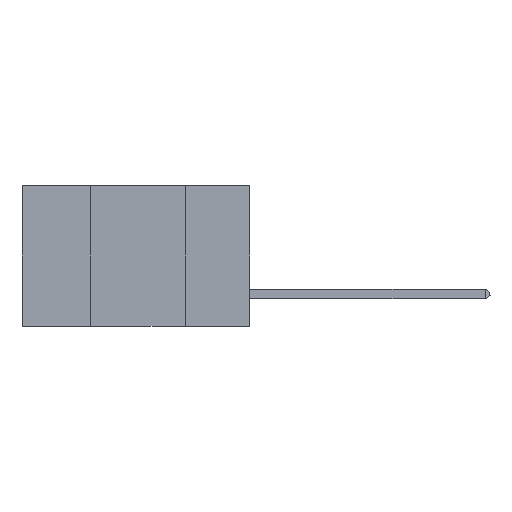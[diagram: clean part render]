
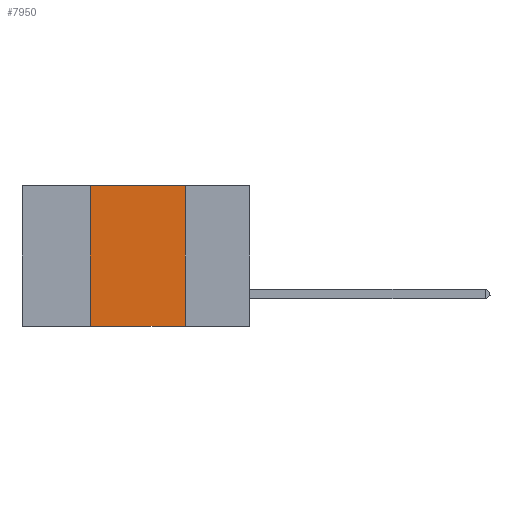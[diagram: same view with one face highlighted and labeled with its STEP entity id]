
A CAD part, left-side view. The second image highlights one B-rep face of the part: STEP entity #7950.
In plain terms, the highlighted planar face has unit normal (-1, 0, 0).
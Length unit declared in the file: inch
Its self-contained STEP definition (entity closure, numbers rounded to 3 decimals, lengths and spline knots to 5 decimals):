
#810 = VECTOR ( 'NONE', #14395, 39.37008 ) ;
#1160 = ORIENTED_EDGE ( 'NONE', *, *, #2776, .F. ) ;
#1202 = EDGE_CURVE ( 'NONE', #4131, #8091, #5164, .T. ) ;
#1248 = DIRECTION ( 'NONE',  ( 0., 0., -1. ) ) ;
#1480 = CARTESIAN_POINT ( 'NONE',  ( 0., 0.42, -0.37 ) ) ;
#2776 = EDGE_CURVE ( 'NONE', #8091, #14675, #6530, .T. ) ;
#3231 = ORIENTED_EDGE ( 'NONE', *, *, #1202, .F. ) ;
#3407 = PLANE ( 'NONE',  #6758 ) ;
#4131 = VERTEX_POINT ( 'NONE', #1480 ) ;
#4232 = CARTESIAN_POINT ( 'NONE',  ( 0., 0.42, 0. ) ) ;
#4282 = DIRECTION ( 'NONE',  ( 0., -1., 0. ) ) ;
#4683 = VECTOR ( 'NONE', #1248, 39.37008 ) ;
#5164 = LINE ( 'NONE', #4232, #810 ) ;
#6530 = LINE ( 'NONE', #12232, #15774 ) ;
#6758 = AXIS2_PLACEMENT_3D ( 'NONE', #12238, #14781, #8501 ) ;
#7152 = VECTOR ( 'NONE', #4282, 39.37008 ) ;
#7477 = CARTESIAN_POINT ( 'NONE',  ( 0., 0.17, -0.37 ) ) ;
#7607 = EDGE_CURVE ( 'NONE', #4131, #9351, #8154, .T. ) ;
#7641 = CARTESIAN_POINT ( 'NONE',  ( 0., 0.17, 0. ) ) ;
#7950 = ADVANCED_FACE ( 'NONE', ( #13291 ), #3407, .F. ) ;
#8091 = VERTEX_POINT ( 'NONE', #8616 ) ;
#8154 = LINE ( 'NONE', #13505, #7152 ) ;
#8501 = DIRECTION ( 'NONE',  ( 0., 0., -1. ) ) ;
#8502 = EDGE_LOOP ( 'NONE', ( #13653, #1160, #3231, #13175 ) ) ;
#8616 = CARTESIAN_POINT ( 'NONE',  ( 0., 0.42, 0. ) ) ;
#9351 = VERTEX_POINT ( 'NONE', #7477 ) ;
#9645 = LINE ( 'NONE', #7641, #4683 ) ;
#12232 = CARTESIAN_POINT ( 'NONE',  ( 0., 0.6, 0. ) ) ;
#12238 = CARTESIAN_POINT ( 'NONE',  ( 0., 0.6, 0. ) ) ;
#12406 = DIRECTION ( 'NONE',  ( 0., -1., 0. ) ) ;
#13175 = ORIENTED_EDGE ( 'NONE', *, *, #7607, .T. ) ;
#13291 = FACE_OUTER_BOUND ( 'NONE', #8502, .T. ) ;
#13505 = CARTESIAN_POINT ( 'NONE',  ( 0., 0.6, -0.37 ) ) ;
#13653 = ORIENTED_EDGE ( 'NONE', *, *, #16226, .F. ) ;
#14395 = DIRECTION ( 'NONE',  ( 0., 0., 1. ) ) ;
#14675 = VERTEX_POINT ( 'NONE', #14865 ) ;
#14781 = DIRECTION ( 'NONE',  ( 1., 0., 0. ) ) ;
#14865 = CARTESIAN_POINT ( 'NONE',  ( 0., 0.17, 0. ) ) ;
#15774 = VECTOR ( 'NONE', #12406, 39.37008 ) ;
#16226 = EDGE_CURVE ( 'NONE', #14675, #9351, #9645, .T. ) ;
